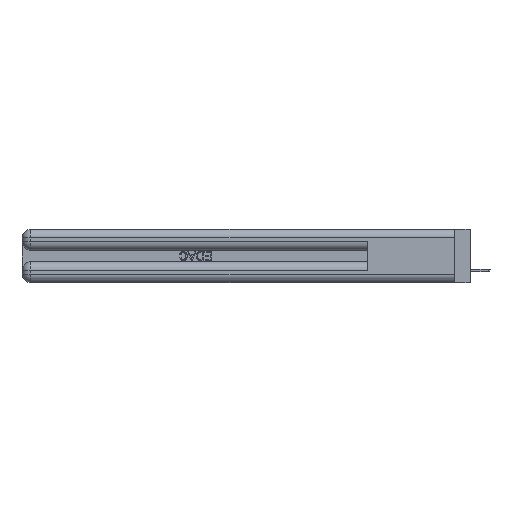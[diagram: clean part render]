
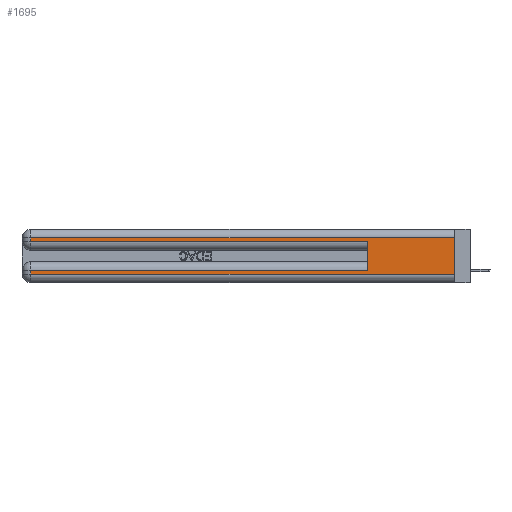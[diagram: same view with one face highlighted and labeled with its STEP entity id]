
A CAD part, left-side view. The second image highlights one B-rep face of the part: STEP entity #1695.
In plain terms, the highlighted planar face has unit normal (-1, 0, 0).
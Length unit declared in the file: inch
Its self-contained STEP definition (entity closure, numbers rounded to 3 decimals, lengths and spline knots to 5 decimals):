
#58 = DIRECTION ( 'NONE',  ( 0., 0., -1. ) ) ;
#1688 = LINE ( 'NONE', #9029, #45849 ) ;
#1695 = ADVANCED_FACE ( 'NONE', ( #34623 ), #27739, .F. ) ;
#3256 = DIRECTION ( 'NONE',  ( 0., 0., 1. ) ) ;
#3774 = VECTOR ( 'NONE', #10832, 39.37008 ) ;
#3847 = LINE ( 'NONE', #29213, #25148 ) ;
#4069 = LINE ( 'NONE', #25634, #31995 ) ;
#4211 = DIRECTION ( 'NONE',  ( 0., -1., 0. ) ) ;
#4772 = EDGE_CURVE ( 'NONE', #40029, #40040, #29796, .T. ) ;
#6228 = ORIENTED_EDGE ( 'NONE', *, *, #44311, .T. ) ;
#7720 = EDGE_CURVE ( 'NONE', #22471, #40029, #3847, .T. ) ;
#9029 = CARTESIAN_POINT ( 'NONE',  ( 0., 0., 0.085 ) ) ;
#9887 = CARTESIAN_POINT ( 'NONE',  ( 0., 2.94, 0.285 ) ) ;
#10051 = LINE ( 'NONE', #31608, #31716 ) ;
#10215 = DIRECTION ( 'NONE',  ( 0., -1., 0. ) ) ;
#10294 = CARTESIAN_POINT ( 'NONE',  ( 0., 2.94, 0.085 ) ) ;
#10724 = DIRECTION ( 'NONE',  ( 0., 1., 0. ) ) ;
#10832 = DIRECTION ( 'NONE',  ( 0., 0., -1. ) ) ;
#11964 = EDGE_CURVE ( 'NONE', #35039, #35027, #21351, .T. ) ;
#12291 = VECTOR ( 'NONE', #10215, 39.37008 ) ;
#13162 = ORIENTED_EDGE ( 'NONE', *, *, #7720, .T. ) ;
#14241 = CARTESIAN_POINT ( 'NONE',  ( 0., 2.94, 0.06 ) ) ;
#15922 = ORIENTED_EDGE ( 'NONE', *, *, #11964, .T. ) ;
#16377 = DIRECTION ( 'NONE',  ( 0., 0., -1. ) ) ;
#17483 = ORIENTED_EDGE ( 'NONE', *, *, #26932, .F. ) ;
#18249 = CARTESIAN_POINT ( 'NONE',  ( 0., 0., 0.31 ) ) ;
#19218 = EDGE_LOOP ( 'NONE', ( #17483, #6228, #13162, #20635, #33525, #32509, #29632, #15922 ) ) ;
#20635 = ORIENTED_EDGE ( 'NONE', *, *, #4772, .T. ) ;
#21351 = LINE ( 'NONE', #32244, #12291 ) ;
#22183 = VECTOR ( 'NONE', #3256, 39.37008 ) ;
#22471 = VERTEX_POINT ( 'NONE', #24327 ) ;
#24218 = EDGE_CURVE ( 'NONE', #40706, #35039, #10051, .T. ) ;
#24327 = CARTESIAN_POINT ( 'NONE',  ( 0., 2.94, 0.31 ) ) ;
#25050 = CARTESIAN_POINT ( 'NONE',  ( 0., 0.6, 0.145 ) ) ;
#25148 = VECTOR ( 'NONE', #58, 39.37008 ) ;
#25634 = CARTESIAN_POINT ( 'NONE',  ( 0., 0., 0.31 ) ) ;
#26932 = EDGE_CURVE ( 'NONE', #33137, #35027, #44028, .T. ) ;
#27185 = CARTESIAN_POINT ( 'NONE',  ( 0., 0.6, 0.285 ) ) ;
#27405 = VECTOR ( 'NONE', #4211, 39.37008 ) ;
#27739 = PLANE ( 'NONE',  #34000 ) ;
#29213 = CARTESIAN_POINT ( 'NONE',  ( 0., 2.94, 0.37 ) ) ;
#29632 = ORIENTED_EDGE ( 'NONE', *, *, #24218, .T. ) ;
#29796 = LINE ( 'NONE', #36926, #27405 ) ;
#30596 = DIRECTION ( 'NONE',  ( 0., 1., 0. ) ) ;
#30610 = EDGE_CURVE ( 'NONE', #34879, #40040, #46904, .T. ) ;
#31072 = CARTESIAN_POINT ( 'NONE',  ( 0., 0.6, 0.085 ) ) ;
#31382 = DIRECTION ( 'NONE',  ( 0., 0., -1. ) ) ;
#31608 = CARTESIAN_POINT ( 'NONE',  ( 0., 2.94, 0.37 ) ) ;
#31716 = VECTOR ( 'NONE', #31382, 39.37008 ) ;
#31995 = VECTOR ( 'NONE', #10724, 39.37008 ) ;
#32244 = CARTESIAN_POINT ( 'NONE',  ( 0., 0., 0.06 ) ) ;
#32509 = ORIENTED_EDGE ( 'NONE', *, *, #34974, .T. ) ;
#33137 = VERTEX_POINT ( 'NONE', #18249 ) ;
#33322 = CARTESIAN_POINT ( 'NONE',  ( 0., 0., 0.37 ) ) ;
#33525 = ORIENTED_EDGE ( 'NONE', *, *, #30610, .F. ) ;
#34000 = AXIS2_PLACEMENT_3D ( 'NONE', #42236, #37723, #16377 ) ;
#34623 = FACE_OUTER_BOUND ( 'NONE', #19218, .T. ) ;
#34879 = VERTEX_POINT ( 'NONE', #31072 ) ;
#34974 = EDGE_CURVE ( 'NONE', #34879, #40706, #1688, .T. ) ;
#35027 = VERTEX_POINT ( 'NONE', #42957 ) ;
#35039 = VERTEX_POINT ( 'NONE', #14241 ) ;
#36926 = CARTESIAN_POINT ( 'NONE',  ( 0., 0., 0.285 ) ) ;
#37723 = DIRECTION ( 'NONE',  ( 1., 0., 0. ) ) ;
#40029 = VERTEX_POINT ( 'NONE', #9887 ) ;
#40040 = VERTEX_POINT ( 'NONE', #27185 ) ;
#40706 = VERTEX_POINT ( 'NONE', #10294 ) ;
#42236 = CARTESIAN_POINT ( 'NONE',  ( 0., 0., 0.37 ) ) ;
#42957 = CARTESIAN_POINT ( 'NONE',  ( 0., 0., 0.06 ) ) ;
#44028 = LINE ( 'NONE', #33322, #3774 ) ;
#44311 = EDGE_CURVE ( 'NONE', #33137, #22471, #4069, .T. ) ;
#45849 = VECTOR ( 'NONE', #30596, 39.37008 ) ;
#46904 = LINE ( 'NONE', #25050, #22183 ) ;
